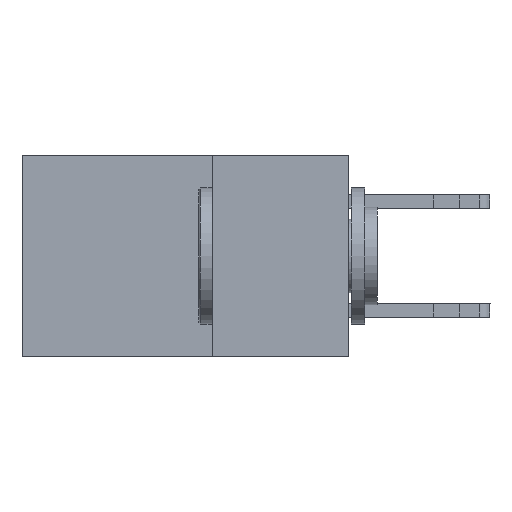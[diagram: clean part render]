
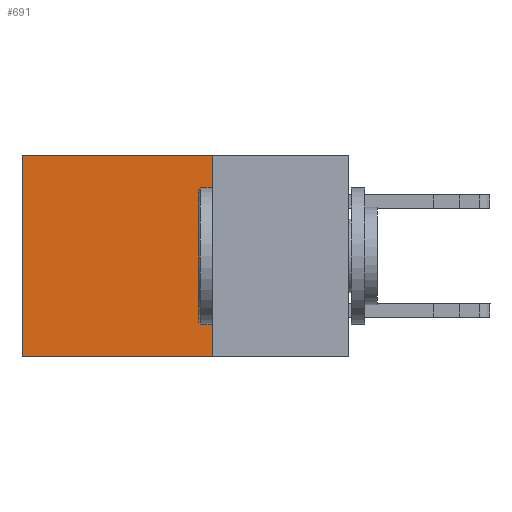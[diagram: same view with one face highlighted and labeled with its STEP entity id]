
A CAD part, left-side view. The second image highlights one B-rep face of the part: STEP entity #691.
In plain terms, the highlighted planar face has unit normal (-1, 0, 0).
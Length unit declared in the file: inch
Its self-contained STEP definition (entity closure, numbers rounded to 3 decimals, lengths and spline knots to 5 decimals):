
#185 = LINE ( 'NONE', #5897, #695 ) ;
#440 = EDGE_CURVE ( 'NONE', #8114, #2094, #2583, .T. ) ;
#482 = ORIENTED_EDGE ( 'NONE', *, *, #7055, .T. ) ;
#691 = ADVANCED_FACE ( 'NONE', ( #4799 ), #917, .F. ) ;
#695 = VECTOR ( 'NONE', #6620, 39.37008 ) ;
#697 = CARTESIAN_POINT ( 'NONE',  ( 0.2615, 0.25, 0. ) ) ;
#917 = PLANE ( 'NONE',  #6571 ) ;
#1063 = VERTEX_POINT ( 'NONE', #10235 ) ;
#1196 = CARTESIAN_POINT ( 'NONE',  ( 0.2615, 0.6, 0. ) ) ;
#1298 = VERTEX_POINT ( 'NONE', #5466 ) ;
#1607 = EDGE_CURVE ( 'NONE', #1063, #2094, #6963, .T. ) ;
#1991 = LINE ( 'NONE', #697, #8302 ) ;
#2094 = VERTEX_POINT ( 'NONE', #4052 ) ;
#2390 = DIRECTION ( 'NONE',  ( 0., 1., 0. ) ) ;
#2420 = ORIENTED_EDGE ( 'NONE', *, *, #1607, .F. ) ;
#2566 = VECTOR ( 'NONE', #5495, 39.37008 ) ;
#2583 = LINE ( 'NONE', #10371, #4160 ) ;
#4052 = CARTESIAN_POINT ( 'NONE',  ( 0.2615, 0.6, -0.37 ) ) ;
#4160 = VECTOR ( 'NONE', #4578, 39.37008 ) ;
#4578 = DIRECTION ( 'NONE',  ( 0., 0., -1. ) ) ;
#4799 = FACE_OUTER_BOUND ( 'NONE', #6925, .T. ) ;
#5032 = DIRECTION ( 'NONE',  ( 0., 0., -1. ) ) ;
#5466 = CARTESIAN_POINT ( 'NONE',  ( 0.2615, 0.25, 0. ) ) ;
#5495 = DIRECTION ( 'NONE',  ( 0., 1., 0. ) ) ;
#5557 = CARTESIAN_POINT ( 'NONE',  ( 0.2615, 0.25, -0.37 ) ) ;
#5897 = CARTESIAN_POINT ( 'NONE',  ( 0.2615, 0.25, -0.37 ) ) ;
#6571 = AXIS2_PLACEMENT_3D ( 'NONE', #9127, #9965, #5032 ) ;
#6620 = DIRECTION ( 'NONE',  ( 0., 0., -1. ) ) ;
#6925 = EDGE_LOOP ( 'NONE', ( #10076, #2420, #7892, #482 ) ) ;
#6963 = LINE ( 'NONE', #5557, #2566 ) ;
#7055 = EDGE_CURVE ( 'NONE', #1298, #8114, #1991, .T. ) ;
#7892 = ORIENTED_EDGE ( 'NONE', *, *, #8502, .F. ) ;
#8114 = VERTEX_POINT ( 'NONE', #1196 ) ;
#8302 = VECTOR ( 'NONE', #2390, 39.37008 ) ;
#8502 = EDGE_CURVE ( 'NONE', #1298, #1063, #185, .T. ) ;
#9127 = CARTESIAN_POINT ( 'NONE',  ( 0.2615, 0.25, -0.37 ) ) ;
#9965 = DIRECTION ( 'NONE',  ( 1., 0., 0. ) ) ;
#10076 = ORIENTED_EDGE ( 'NONE', *, *, #440, .T. ) ;
#10235 = CARTESIAN_POINT ( 'NONE',  ( 0.2615, 0.25, -0.37 ) ) ;
#10371 = CARTESIAN_POINT ( 'NONE',  ( 0.2615, 0.6, -0.37 ) ) ;
